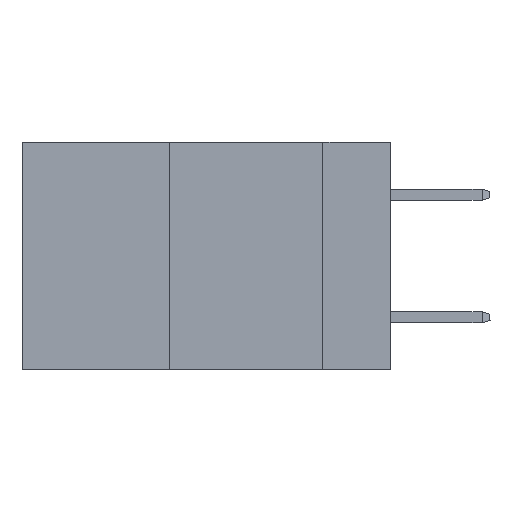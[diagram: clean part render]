
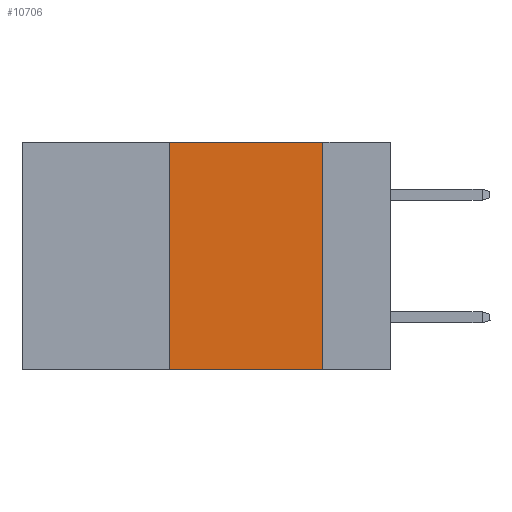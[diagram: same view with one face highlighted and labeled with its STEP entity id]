
A CAD part, left-side view. The second image highlights one B-rep face of the part: STEP entity #10706.
In plain terms, the highlighted planar face has unit normal (-1, 0, 0).
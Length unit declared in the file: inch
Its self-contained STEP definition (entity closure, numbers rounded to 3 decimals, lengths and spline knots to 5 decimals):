
#247 = CARTESIAN_POINT ( 'NONE',  ( 0., 0.6, -0.37 ) ) ;
#261 = DIRECTION ( 'NONE',  ( 0., 0., -1. ) ) ;
#1113 = EDGE_CURVE ( 'NONE', #24052, #17764, #12210, .T. ) ;
#2176 = DIRECTION ( 'NONE',  ( 0., 0., 1. ) ) ;
#2514 = ORIENTED_EDGE ( 'NONE', *, *, #1113, .F. ) ;
#4837 = EDGE_CURVE ( 'NONE', #14697, #14880, #7913, .T. ) ;
#5224 = VECTOR ( 'NONE', #22767, 39.37008 ) ;
#5762 = FACE_OUTER_BOUND ( 'NONE', #16554, .T. ) ;
#6787 = DIRECTION ( 'NONE',  ( 0., -1., 0. ) ) ;
#7913 = LINE ( 'NONE', #13587, #17981 ) ;
#8357 = CARTESIAN_POINT ( 'NONE',  ( 0., 0.36, -0.37 ) ) ;
#9927 = ORIENTED_EDGE ( 'NONE', *, *, #4837, .F. ) ;
#10044 = DIRECTION ( 'NONE',  ( 0., 0., -1. ) ) ;
#10706 = ADVANCED_FACE ( 'NONE', ( #5762 ), #20242, .F. ) ;
#11333 = CARTESIAN_POINT ( 'NONE',  ( 0., 0.11, 0. ) ) ;
#12210 = LINE ( 'NONE', #12332, #22427 ) ;
#12332 = CARTESIAN_POINT ( 'NONE',  ( 0., 0.36, 0. ) ) ;
#13587 = CARTESIAN_POINT ( 'NONE',  ( 0., 0.11, 0. ) ) ;
#14697 = VERTEX_POINT ( 'NONE', #11333 ) ;
#14744 = ORIENTED_EDGE ( 'NONE', *, *, #22354, .F. ) ;
#14880 = VERTEX_POINT ( 'NONE', #18706 ) ;
#15654 = ORIENTED_EDGE ( 'NONE', *, *, #23475, .T. ) ;
#15951 = DIRECTION ( 'NONE',  ( 1., 0., 0. ) ) ;
#16074 = LINE ( 'NONE', #247, #5224 ) ;
#16438 = AXIS2_PLACEMENT_3D ( 'NONE', #20111, #15951, #261 ) ;
#16554 = EDGE_LOOP ( 'NONE', ( #9927, #14744, #2514, #15654 ) ) ;
#16991 = LINE ( 'NONE', #25292, #21043 ) ;
#17764 = VERTEX_POINT ( 'NONE', #25543 ) ;
#17981 = VECTOR ( 'NONE', #10044, 39.37008 ) ;
#18706 = CARTESIAN_POINT ( 'NONE',  ( 0., 0.11, -0.37 ) ) ;
#20111 = CARTESIAN_POINT ( 'NONE',  ( 0., 0.6, 0. ) ) ;
#20242 = PLANE ( 'NONE',  #16438 ) ;
#21043 = VECTOR ( 'NONE', #6787, 39.37008 ) ;
#22354 = EDGE_CURVE ( 'NONE', #17764, #14697, #16991, .T. ) ;
#22427 = VECTOR ( 'NONE', #2176, 39.37008 ) ;
#22767 = DIRECTION ( 'NONE',  ( 0., -1., 0. ) ) ;
#23475 = EDGE_CURVE ( 'NONE', #24052, #14880, #16074, .T. ) ;
#24052 = VERTEX_POINT ( 'NONE', #8357 ) ;
#25292 = CARTESIAN_POINT ( 'NONE',  ( 0., 0.6, 0. ) ) ;
#25543 = CARTESIAN_POINT ( 'NONE',  ( 0., 0.36, 0. ) ) ;
